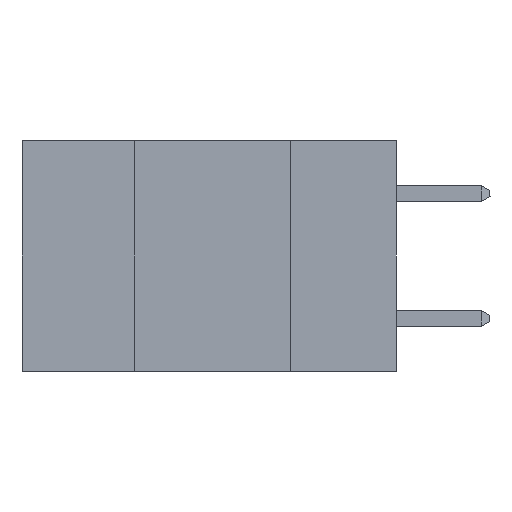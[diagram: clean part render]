
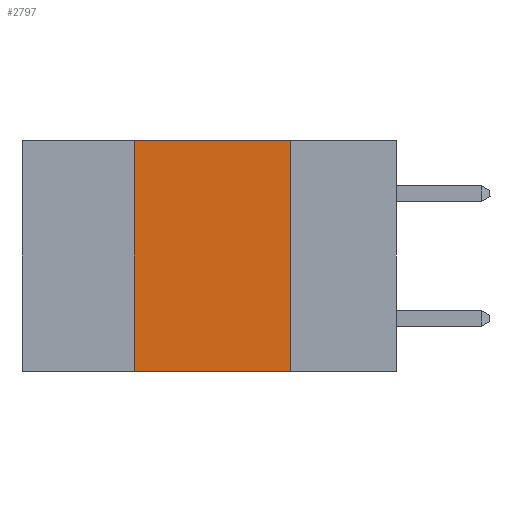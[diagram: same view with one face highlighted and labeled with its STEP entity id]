
A CAD part, left-side view. The second image highlights one B-rep face of the part: STEP entity #2797.
In plain terms, the highlighted planar face has unit normal (-1, 0, 0).
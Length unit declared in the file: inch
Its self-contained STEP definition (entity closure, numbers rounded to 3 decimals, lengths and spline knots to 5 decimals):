
#198 = VECTOR ( 'NONE', #10568, 39.37008 ) ;
#745 = CARTESIAN_POINT ( 'NONE',  ( 0., 0.42, 0. ) ) ;
#1058 = ORIENTED_EDGE ( 'NONE', *, *, #9469, .F. ) ;
#1555 = LINE ( 'NONE', #10236, #5238 ) ;
#2238 = EDGE_CURVE ( 'NONE', #9308, #7828, #1555, .T. ) ;
#2313 = PLANE ( 'NONE',  #5297 ) ;
#2543 = LINE ( 'NONE', #4662, #5607 ) ;
#2797 = ADVANCED_FACE ( 'NONE', ( #6441 ), #2313, .F. ) ;
#3460 = CARTESIAN_POINT ( 'NONE',  ( 0., 0.42, 0. ) ) ;
#4365 = CARTESIAN_POINT ( 'NONE',  ( 0., 0.17, -0.37 ) ) ;
#4541 = ORIENTED_EDGE ( 'NONE', *, *, #2238, .T. ) ;
#4662 = CARTESIAN_POINT ( 'NONE',  ( 0., 0.17, 0. ) ) ;
#4705 = DIRECTION ( 'NONE',  ( 0., 0., -1. ) ) ;
#5013 = CARTESIAN_POINT ( 'NONE',  ( 0., 0.6, 0. ) ) ;
#5192 = CARTESIAN_POINT ( 'NONE',  ( 0., 0.6, 0. ) ) ;
#5234 = DIRECTION ( 'NONE',  ( 1., 0., 0. ) ) ;
#5238 = VECTOR ( 'NONE', #7245, 39.37008 ) ;
#5297 = AXIS2_PLACEMENT_3D ( 'NONE', #5192, #5234, #12230 ) ;
#5607 = VECTOR ( 'NONE', #4705, 39.37008 ) ;
#5845 = VECTOR ( 'NONE', #9903, 39.37008 ) ;
#6441 = FACE_OUTER_BOUND ( 'NONE', #8105, .T. ) ;
#6473 = LINE ( 'NONE', #5013, #5845 ) ;
#7245 = DIRECTION ( 'NONE',  ( 0., -1., 0. ) ) ;
#7387 = CARTESIAN_POINT ( 'NONE',  ( 0., 0.17, 0. ) ) ;
#7825 = VERTEX_POINT ( 'NONE', #3460 ) ;
#7828 = VERTEX_POINT ( 'NONE', #4365 ) ;
#8105 = EDGE_LOOP ( 'NONE', ( #1058, #12067, #11533, #4541 ) ) ;
#9308 = VERTEX_POINT ( 'NONE', #9409 ) ;
#9409 = CARTESIAN_POINT ( 'NONE',  ( 0., 0.42, -0.37 ) ) ;
#9469 = EDGE_CURVE ( 'NONE', #11862, #7828, #2543, .T. ) ;
#9903 = DIRECTION ( 'NONE',  ( 0., -1., 0. ) ) ;
#10236 = CARTESIAN_POINT ( 'NONE',  ( 0., 0.6, -0.37 ) ) ;
#10568 = DIRECTION ( 'NONE',  ( 0., 0., 1. ) ) ;
#11074 = LINE ( 'NONE', #745, #198 ) ;
#11207 = EDGE_CURVE ( 'NONE', #9308, #7825, #11074, .T. ) ;
#11365 = EDGE_CURVE ( 'NONE', #7825, #11862, #6473, .T. ) ;
#11533 = ORIENTED_EDGE ( 'NONE', *, *, #11207, .F. ) ;
#11862 = VERTEX_POINT ( 'NONE', #7387 ) ;
#12067 = ORIENTED_EDGE ( 'NONE', *, *, #11365, .F. ) ;
#12230 = DIRECTION ( 'NONE',  ( 0., 0., -1. ) ) ;
